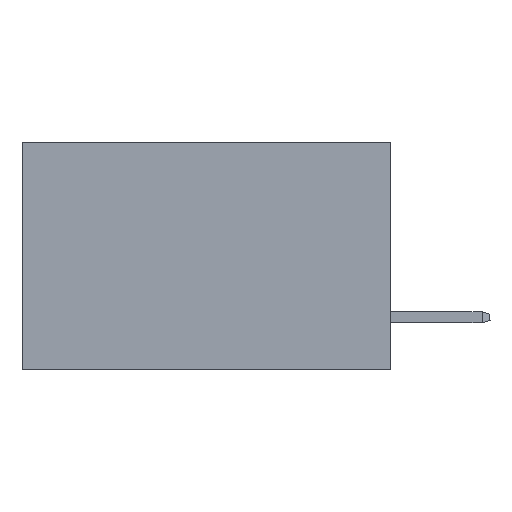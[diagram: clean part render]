
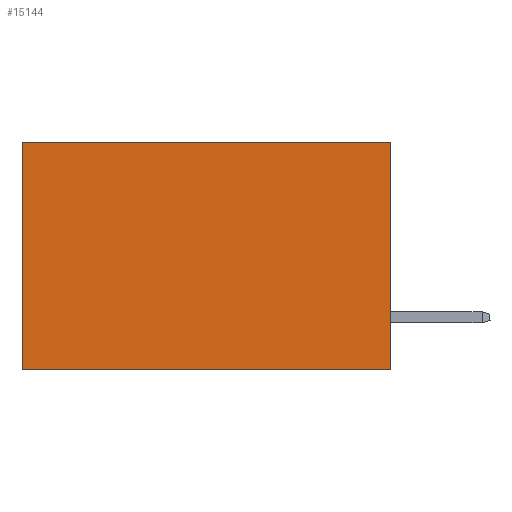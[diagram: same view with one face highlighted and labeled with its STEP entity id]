
A CAD part, left-side view. The second image highlights one B-rep face of the part: STEP entity #15144.
In plain terms, the highlighted planar face has unit normal (-1, 0, 0).
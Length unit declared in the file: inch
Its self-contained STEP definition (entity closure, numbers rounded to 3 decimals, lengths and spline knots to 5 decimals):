
#396 = LINE ( 'NONE', #6159, #16523 ) ;
#565 = CARTESIAN_POINT ( 'NONE',  ( 0.2875, 0., 0. ) ) ;
#1037 = AXIS2_PLACEMENT_3D ( 'NONE', #14639, #17524, #11283 ) ;
#1171 = EDGE_CURVE ( 'NONE', #19773, #14727, #396, .T. ) ;
#1825 = PLANE ( 'NONE',  #1037 ) ;
#2002 = FACE_OUTER_BOUND ( 'NONE', #3748, .T. ) ;
#2018 = DIRECTION ( 'NONE',  ( 0., 1., 0. ) ) ;
#2965 = ORIENTED_EDGE ( 'NONE', *, *, #1171, .T. ) ;
#3748 = EDGE_LOOP ( 'NONE', ( #2965, #10721, #5618, #5036 ) ) ;
#4695 = LINE ( 'NONE', #16244, #7349 ) ;
#5036 = ORIENTED_EDGE ( 'NONE', *, *, #16500, .T. ) ;
#5618 = ORIENTED_EDGE ( 'NONE', *, *, #8508, .F. ) ;
#5780 = CARTESIAN_POINT ( 'NONE',  ( 0.2875, 0., -0.37 ) ) ;
#6134 = LINE ( 'NONE', #6943, #7799 ) ;
#6159 = CARTESIAN_POINT ( 'NONE',  ( 0.2875, 0.6, 0. ) ) ;
#6943 = CARTESIAN_POINT ( 'NONE',  ( 0.2875, 0., -0.37 ) ) ;
#7349 = VECTOR ( 'NONE', #9885, 39.37008 ) ;
#7799 = VECTOR ( 'NONE', #2018, 39.37008 ) ;
#7861 = EDGE_CURVE ( 'NONE', #13180, #14727, #6134, .T. ) ;
#8508 = EDGE_CURVE ( 'NONE', #12552, #13180, #18319, .T. ) ;
#9885 = DIRECTION ( 'NONE',  ( 0., 1., 0. ) ) ;
#10721 = ORIENTED_EDGE ( 'NONE', *, *, #7861, .F. ) ;
#11283 = DIRECTION ( 'NONE',  ( 0., 0., -1. ) ) ;
#12065 = CARTESIAN_POINT ( 'NONE',  ( 0.2875, 0.6, 0. ) ) ;
#12552 = VERTEX_POINT ( 'NONE', #20224 ) ;
#13180 = VERTEX_POINT ( 'NONE', #5780 ) ;
#14639 = CARTESIAN_POINT ( 'NONE',  ( 0.2875, 0., 0. ) ) ;
#14727 = VERTEX_POINT ( 'NONE', #16008 ) ;
#15144 = ADVANCED_FACE ( 'NONE', ( #2002 ), #1825, .F. ) ;
#16008 = CARTESIAN_POINT ( 'NONE',  ( 0.2875, 0.6, -0.37 ) ) ;
#16244 = CARTESIAN_POINT ( 'NONE',  ( 0.2875, 0., 0. ) ) ;
#16500 = EDGE_CURVE ( 'NONE', #12552, #19773, #4695, .T. ) ;
#16523 = VECTOR ( 'NONE', #18863, 39.37008 ) ;
#17524 = DIRECTION ( 'NONE',  ( 1., 0., 0. ) ) ;
#17907 = DIRECTION ( 'NONE',  ( 0., 0., -1. ) ) ;
#18319 = LINE ( 'NONE', #565, #19551 ) ;
#18863 = DIRECTION ( 'NONE',  ( 0., 0., -1. ) ) ;
#19551 = VECTOR ( 'NONE', #17907, 39.37008 ) ;
#19773 = VERTEX_POINT ( 'NONE', #12065 ) ;
#20224 = CARTESIAN_POINT ( 'NONE',  ( 0.2875, 0., 0. ) ) ;
